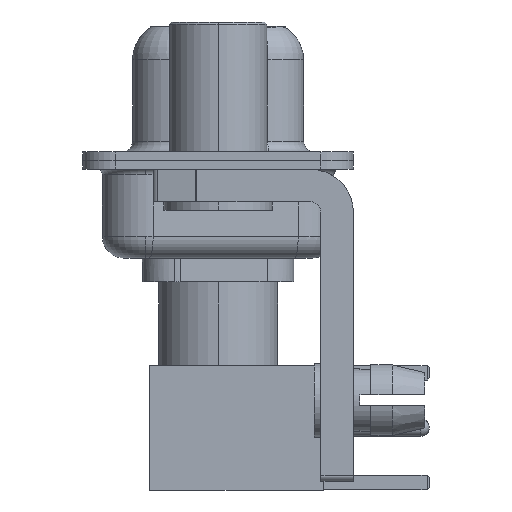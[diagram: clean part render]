
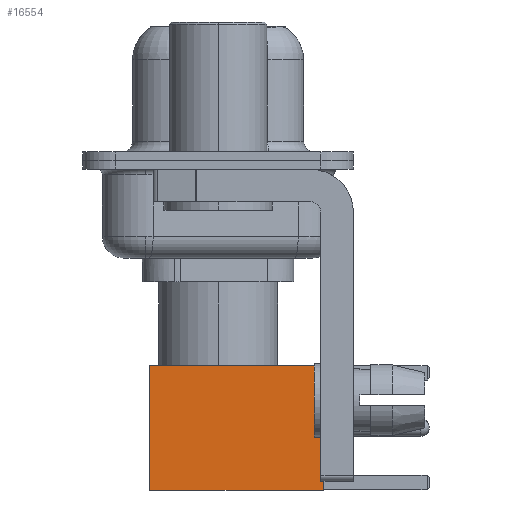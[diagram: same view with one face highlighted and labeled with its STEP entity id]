
A CAD part, left-side view. The second image highlights one B-rep face of the part: STEP entity #16554.
In plain terms, the highlighted face is planar.
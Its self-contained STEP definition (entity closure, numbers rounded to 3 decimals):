
#2338 = VECTOR ( 'NONE', #17207, 1000. ) ;
#2536 = LINE ( 'NONE', #14647, #4122 ) ;
#4122 = VECTOR ( 'NONE', #8727, 1000. ) ;
#4656 = VERTEX_POINT ( 'NONE', #5576 ) ;
#4823 = ORIENTED_EDGE ( 'NONE', *, *, #16779, .F. ) ;
#5576 = CARTESIAN_POINT ( 'NONE',  ( -2.875, 2.875, 8. ) ) ;
#5614 = EDGE_LOOP ( 'NONE', ( #10808, #22274, #4823, #19209 ) ) ;
#5849 = LINE ( 'NONE', #20136, #13451 ) ;
#7772 = CARTESIAN_POINT ( 'NONE',  ( 2.875, 2.875, 8. ) ) ;
#8557 = CARTESIAN_POINT ( 'NONE',  ( 2.875, 2.875, 0. ) ) ;
#8727 = DIRECTION ( 'NONE',  ( 0., 0., -1. ) ) ;
#8790 = VERTEX_POINT ( 'NONE', #8557 ) ;
#9616 = AXIS2_PLACEMENT_3D ( 'NONE', #11486, #11260, #20206 ) ;
#9818 = EDGE_CURVE ( 'NONE', #8790, #16797, #5849, .T. ) ;
#10808 = ORIENTED_EDGE ( 'NONE', *, *, #15434, .T. ) ;
#11260 = DIRECTION ( 'NONE',  ( 0., 1., 0. ) ) ;
#11486 = CARTESIAN_POINT ( 'NONE',  ( 2.875, 2.875, 0. ) ) ;
#13451 = VECTOR ( 'NONE', #19682, 1000. ) ;
#14647 = CARTESIAN_POINT ( 'NONE',  ( 2.875, 2.875, 0. ) ) ;
#15158 = CARTESIAN_POINT ( 'NONE',  ( -2.875, 2.875, 0. ) ) ;
#15434 = EDGE_CURVE ( 'NONE', #18281, #8790, #2536, .T. ) ;
#15441 = DIRECTION ( 'NONE',  ( -1., 0., 0. ) ) ;
#15774 = EDGE_CURVE ( 'NONE', #18281, #4656, #17606, .T. ) ;
#15945 = CARTESIAN_POINT ( 'NONE',  ( -2.875, 2.875, 0. ) ) ;
#16554 = ADVANCED_FACE ( 'NONE', ( #20316 ), #19974, .T. ) ;
#16779 = EDGE_CURVE ( 'NONE', #4656, #16797, #18936, .T. ) ;
#16797 = VERTEX_POINT ( 'NONE', #15945 ) ;
#17207 = DIRECTION ( 'NONE',  ( 0., 0., -1. ) ) ;
#17606 = LINE ( 'NONE', #18987, #22016 ) ;
#18281 = VERTEX_POINT ( 'NONE', #7772 ) ;
#18936 = LINE ( 'NONE', #15158, #2338 ) ;
#18987 = CARTESIAN_POINT ( 'NONE',  ( 0., 2.875, 8. ) ) ;
#19209 = ORIENTED_EDGE ( 'NONE', *, *, #15774, .F. ) ;
#19682 = DIRECTION ( 'NONE',  ( -1., 0., 0. ) ) ;
#19974 = PLANE ( 'NONE',  #9616 ) ;
#20136 = CARTESIAN_POINT ( 'NONE',  ( 0., 2.875, 0. ) ) ;
#20206 = DIRECTION ( 'NONE',  ( 0., 0., 1. ) ) ;
#20316 = FACE_OUTER_BOUND ( 'NONE', #5614, .T. ) ;
#22016 = VECTOR ( 'NONE', #15441, 1000. ) ;
#22274 = ORIENTED_EDGE ( 'NONE', *, *, #9818, .T. ) ;
